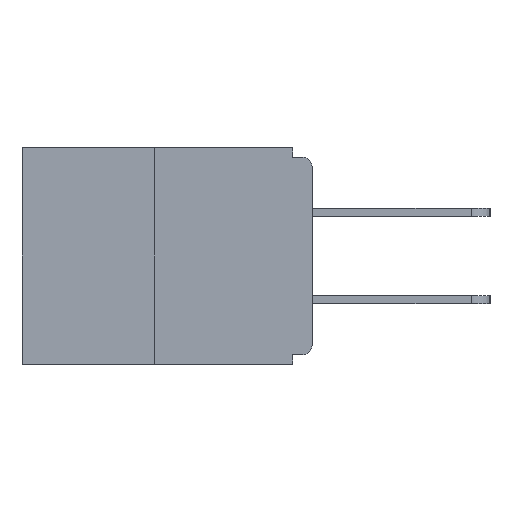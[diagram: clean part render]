
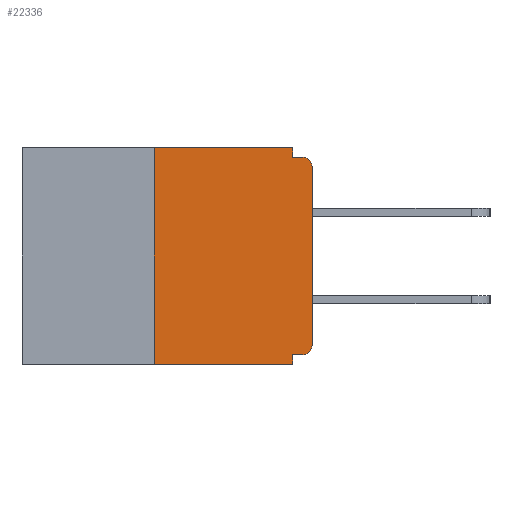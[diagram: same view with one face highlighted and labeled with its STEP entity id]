
A CAD part, left-side view. The second image highlights one B-rep face of the part: STEP entity #22336.
In plain terms, the highlighted planar face has unit normal (-1, 0, 0).
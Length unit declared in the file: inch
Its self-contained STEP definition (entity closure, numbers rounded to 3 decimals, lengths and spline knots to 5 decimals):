
#1240 = DIRECTION ( 'NONE',  ( 0., 0., -1. ) ) ;
#2143 = CARTESIAN_POINT ( 'NONE',  ( 0., 0.25, 0. ) ) ;
#2578 = ORIENTED_EDGE ( 'NONE', *, *, #17581, .T. ) ;
#3106 = DIRECTION ( 'NONE',  ( 0., 0., -1. ) ) ;
#3116 = AXIS2_PLACEMENT_3D ( 'NONE', #14906, #15062, #13081 ) ;
#3146 = AXIS2_PLACEMENT_3D ( 'NONE', #16934, #4625, #3106 ) ;
#3303 = CARTESIAN_POINT ( 'NONE',  ( 0., 0., -0.328 ) ) ;
#3544 = CARTESIAN_POINT ( 'NONE',  ( 0., 0.015, -0.015 ) ) ;
#4060 = ORIENTED_EDGE ( 'NONE', *, *, #22677, .F. ) ;
#4079 = ORIENTED_EDGE ( 'NONE', *, *, #8675, .F. ) ;
#4343 = VERTEX_POINT ( 'NONE', #12917 ) ;
#4401 = CARTESIAN_POINT ( 'NONE',  ( 0., 0.46, -0.343 ) ) ;
#4625 = DIRECTION ( 'NONE',  ( -1., 0., 0. ) ) ;
#4827 = DIRECTION ( 'NONE',  ( 0., 1., 0. ) ) ;
#5448 = LINE ( 'NONE', #3303, #8999 ) ;
#5527 = ORIENTED_EDGE ( 'NONE', *, *, #18749, .T. ) ;
#5602 = CARTESIAN_POINT ( 'NONE',  ( 0., 0.015, -0.328 ) ) ;
#5758 = LINE ( 'NONE', #14483, #8749 ) ;
#5908 = DIRECTION ( 'NONE',  ( 1., 0., 0. ) ) ;
#6477 = CARTESIAN_POINT ( 'NONE',  ( 0., 0.25, 0. ) ) ;
#6756 = VERTEX_POINT ( 'NONE', #3544 ) ;
#6939 = VERTEX_POINT ( 'NONE', #8133 ) ;
#6954 = VERTEX_POINT ( 'NONE', #9880 ) ;
#7391 = EDGE_LOOP ( 'NONE', ( #9893, #4060, #2578, #19385, #4079, #12093, #5527, #10141, #15105, #22241 ) ) ;
#8133 = CARTESIAN_POINT ( 'NONE',  ( 0., 0.031, -0.343 ) ) ;
#8162 = LINE ( 'NONE', #6477, #14470 ) ;
#8200 = CARTESIAN_POINT ( 'NONE',  ( 0., 0., -0.03 ) ) ;
#8675 = EDGE_CURVE ( 'NONE', #18420, #6954, #5448, .T. ) ;
#8749 = VECTOR ( 'NONE', #21636, 39.37008 ) ;
#8868 = CARTESIAN_POINT ( 'NONE',  ( 0., 0.46, 0. ) ) ;
#8999 = VECTOR ( 'NONE', #4827, 39.37008 ) ;
#9659 = CIRCLE ( 'NONE', #3146, 0.015 ) ;
#9813 = EDGE_CURVE ( 'NONE', #18420, #16922, #17743, .T. ) ;
#9880 = CARTESIAN_POINT ( 'NONE',  ( 0., 0.031, -0.328 ) ) ;
#9893 = ORIENTED_EDGE ( 'NONE', *, *, #20288, .F. ) ;
#10141 = ORIENTED_EDGE ( 'NONE', *, *, #11734, .T. ) ;
#10337 = VERTEX_POINT ( 'NONE', #2143 ) ;
#10535 = VECTOR ( 'NONE', #20813, 39.37008 ) ;
#10685 = VECTOR ( 'NONE', #11497, 39.37008 ) ;
#11038 = CARTESIAN_POINT ( 'NONE',  ( 0., 0.46, 0. ) ) ;
#11071 = EDGE_CURVE ( 'NONE', #6954, #6939, #20168, .T. ) ;
#11114 = CARTESIAN_POINT ( 'NONE',  ( 0., 0.25, -0.343 ) ) ;
#11236 = EDGE_CURVE ( 'NONE', #20893, #6756, #14090, .T. ) ;
#11497 = DIRECTION ( 'NONE',  ( 0., -1., 0. ) ) ;
#11734 = EDGE_CURVE ( 'NONE', #15224, #6756, #9659, .T. ) ;
#12082 = VERTEX_POINT ( 'NONE', #11114 ) ;
#12093 = ORIENTED_EDGE ( 'NONE', *, *, #9813, .T. ) ;
#12117 = LINE ( 'NONE', #8868, #17885 ) ;
#12465 = VECTOR ( 'NONE', #1240, 39.37008 ) ;
#12582 = FACE_OUTER_BOUND ( 'NONE', #7391, .T. ) ;
#12812 = CARTESIAN_POINT ( 'NONE',  ( 0., 0.031, -0.015 ) ) ;
#12917 = CARTESIAN_POINT ( 'NONE',  ( 0., 0.031, 0. ) ) ;
#13010 = PLANE ( 'NONE',  #20562 ) ;
#13081 = DIRECTION ( 'NONE',  ( 0., 0., -1. ) ) ;
#13643 = CARTESIAN_POINT ( 'NONE',  ( 0., 0., -0.015 ) ) ;
#14090 = LINE ( 'NONE', #13643, #10535 ) ;
#14122 = CARTESIAN_POINT ( 'NONE',  ( 0., 0., -0.313 ) ) ;
#14221 = DIRECTION ( 'NONE',  ( 0., -1., 0. ) ) ;
#14470 = VECTOR ( 'NONE', #20336, 39.37008 ) ;
#14483 = CARTESIAN_POINT ( 'NONE',  ( 0., 0.031, 0. ) ) ;
#14571 = DIRECTION ( 'NONE',  ( 0., 0., 1. ) ) ;
#14906 = CARTESIAN_POINT ( 'NONE',  ( 0., 0.015, -0.313 ) ) ;
#14934 = LINE ( 'NONE', #19619, #20733 ) ;
#15062 = DIRECTION ( 'NONE',  ( -1., 0., 0. ) ) ;
#15105 = ORIENTED_EDGE ( 'NONE', *, *, #11236, .F. ) ;
#15224 = VERTEX_POINT ( 'NONE', #8200 ) ;
#16922 = VERTEX_POINT ( 'NONE', #14122 ) ;
#16934 = CARTESIAN_POINT ( 'NONE',  ( 0., 0.015, -0.03 ) ) ;
#17093 = EDGE_CURVE ( 'NONE', #4343, #20893, #5758, .T. ) ;
#17581 = EDGE_CURVE ( 'NONE', #12082, #6939, #19453, .T. ) ;
#17743 = CIRCLE ( 'NONE', #3116, 0.015 ) ;
#17885 = VECTOR ( 'NONE', #14221, 39.37008 ) ;
#18152 = DIRECTION ( 'NONE',  ( 0., 0., -1. ) ) ;
#18420 = VERTEX_POINT ( 'NONE', #5602 ) ;
#18749 = EDGE_CURVE ( 'NONE', #16922, #15224, #14934, .T. ) ;
#19385 = ORIENTED_EDGE ( 'NONE', *, *, #11071, .F. ) ;
#19453 = LINE ( 'NONE', #4401, #10685 ) ;
#19619 = CARTESIAN_POINT ( 'NONE',  ( 0., 0., 0. ) ) ;
#20168 = LINE ( 'NONE', #22344, #12465 ) ;
#20288 = EDGE_CURVE ( 'NONE', #10337, #4343, #12117, .T. ) ;
#20336 = DIRECTION ( 'NONE',  ( 0., 0., 1. ) ) ;
#20562 = AXIS2_PLACEMENT_3D ( 'NONE', #11038, #5908, #18152 ) ;
#20733 = VECTOR ( 'NONE', #14571, 39.37008 ) ;
#20813 = DIRECTION ( 'NONE',  ( 0., -1., 0. ) ) ;
#20893 = VERTEX_POINT ( 'NONE', #12812 ) ;
#21636 = DIRECTION ( 'NONE',  ( 0., 0., -1. ) ) ;
#22241 = ORIENTED_EDGE ( 'NONE', *, *, #17093, .F. ) ;
#22336 = ADVANCED_FACE ( 'NONE', ( #12582 ), #13010, .F. ) ;
#22344 = CARTESIAN_POINT ( 'NONE',  ( 0., 0.031, -0.343 ) ) ;
#22677 = EDGE_CURVE ( 'NONE', #12082, #10337, #8162, .T. ) ;
